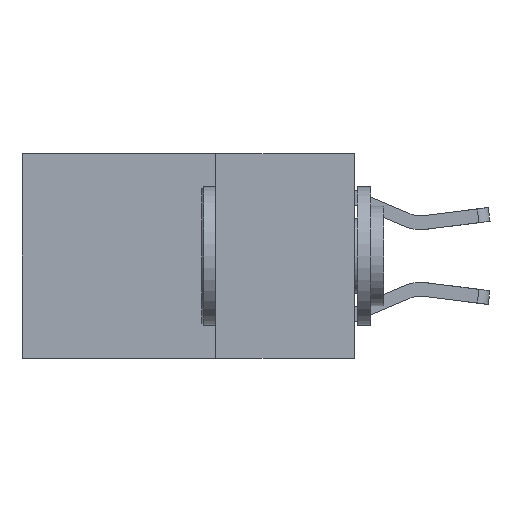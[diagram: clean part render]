
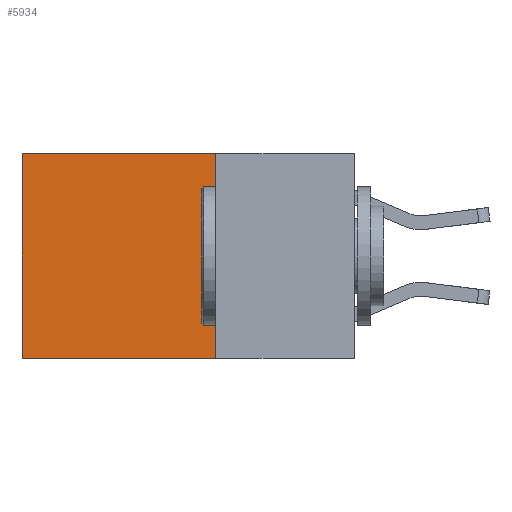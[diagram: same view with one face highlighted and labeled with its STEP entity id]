
A CAD part, left-side view. The second image highlights one B-rep face of the part: STEP entity #5934.
In plain terms, the highlighted planar face has unit normal (-1, 0, 0).
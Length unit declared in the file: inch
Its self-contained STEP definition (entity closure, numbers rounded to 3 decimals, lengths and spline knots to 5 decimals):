
#252 = FACE_OUTER_BOUND ( 'NONE', #3715, .T. ) ;
#443 = CARTESIAN_POINT ( 'NONE',  ( 0.2625, 0.25, 0. ) ) ;
#448 = DIRECTION ( 'NONE',  ( 0., 0., -1. ) ) ;
#714 = VECTOR ( 'NONE', #448, 39.37008 ) ;
#869 = VERTEX_POINT ( 'NONE', #5463 ) ;
#1074 = VECTOR ( 'NONE', #3539, 39.37008 ) ;
#1271 = DIRECTION ( 'NONE',  ( 0., 0., -1. ) ) ;
#2942 = VECTOR ( 'NONE', #1271, 39.37008 ) ;
#2982 = VERTEX_POINT ( 'NONE', #4636 ) ;
#3102 = LINE ( 'NONE', #8314, #714 ) ;
#3202 = CARTESIAN_POINT ( 'NONE',  ( 0.2625, 0.6, 0. ) ) ;
#3209 = EDGE_CURVE ( 'NONE', #869, #2982, #6025, .T. ) ;
#3520 = CARTESIAN_POINT ( 'NONE',  ( 0.2625, 0.25, 0. ) ) ;
#3539 = DIRECTION ( 'NONE',  ( 0., 1., 0. ) ) ;
#3627 = PLANE ( 'NONE',  #7070 ) ;
#3715 = EDGE_LOOP ( 'NONE', ( #10105, #10197, #7528, #8191 ) ) ;
#3996 = EDGE_CURVE ( 'NONE', #7848, #2982, #3102, .T. ) ;
#4284 = VECTOR ( 'NONE', #9768, 39.37008 ) ;
#4425 = EDGE_CURVE ( 'NONE', #5048, #7848, #9748, .T. ) ;
#4636 = CARTESIAN_POINT ( 'NONE',  ( 0.2625, 0.6, -0.37 ) ) ;
#5025 = LINE ( 'NONE', #443, #2942 ) ;
#5048 = VERTEX_POINT ( 'NONE', #5816 ) ;
#5463 = CARTESIAN_POINT ( 'NONE',  ( 0.2625, 0.25, -0.37 ) ) ;
#5816 = CARTESIAN_POINT ( 'NONE',  ( 0.2625, 0.25, 0. ) ) ;
#5934 = ADVANCED_FACE ( 'NONE', ( #252 ), #3627, .F. ) ;
#6025 = LINE ( 'NONE', #7457, #1074 ) ;
#7070 = AXIS2_PLACEMENT_3D ( 'NONE', #9178, #7476, #8280 ) ;
#7457 = CARTESIAN_POINT ( 'NONE',  ( 0.2625, 0.25, -0.37 ) ) ;
#7476 = DIRECTION ( 'NONE',  ( 1., 0., 0. ) ) ;
#7528 = ORIENTED_EDGE ( 'NONE', *, *, #8696, .F. ) ;
#7848 = VERTEX_POINT ( 'NONE', #3202 ) ;
#8191 = ORIENTED_EDGE ( 'NONE', *, *, #4425, .T. ) ;
#8280 = DIRECTION ( 'NONE',  ( 0., 0., -1. ) ) ;
#8314 = CARTESIAN_POINT ( 'NONE',  ( 0.2625, 0.6, 0. ) ) ;
#8696 = EDGE_CURVE ( 'NONE', #5048, #869, #5025, .T. ) ;
#9178 = CARTESIAN_POINT ( 'NONE',  ( 0.2625, 0.25, 0. ) ) ;
#9748 = LINE ( 'NONE', #3520, #4284 ) ;
#9768 = DIRECTION ( 'NONE',  ( 0., 1., 0. ) ) ;
#10105 = ORIENTED_EDGE ( 'NONE', *, *, #3996, .T. ) ;
#10197 = ORIENTED_EDGE ( 'NONE', *, *, #3209, .F. ) ;
